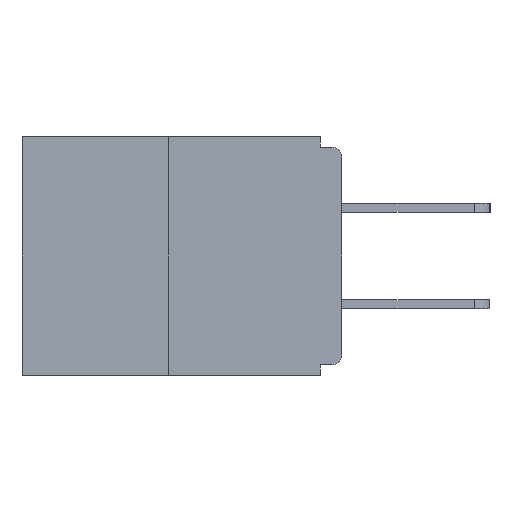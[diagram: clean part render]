
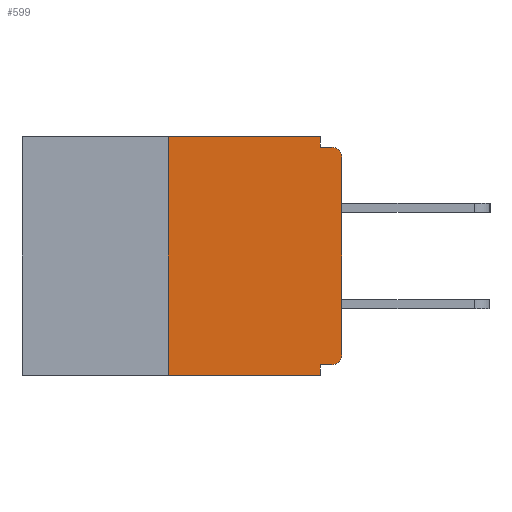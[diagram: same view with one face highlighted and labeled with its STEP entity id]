
A CAD part, left-side view. The second image highlights one B-rep face of the part: STEP entity #599.
In plain terms, the highlighted planar face has unit normal (-1, 0, 0).
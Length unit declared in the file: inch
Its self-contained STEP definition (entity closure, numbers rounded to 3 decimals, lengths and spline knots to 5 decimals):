
#55 = CARTESIAN_POINT ( 'NONE',  ( 0., 0.25, -0.343 ) ) ;
#145 = DIRECTION ( 'NONE',  ( 0., 0., -1. ) ) ;
#154 = LINE ( 'NONE', #9585, #1045 ) ;
#329 = CARTESIAN_POINT ( 'NONE',  ( 0., 0.031, -0.328 ) ) ;
#599 = ADVANCED_FACE ( 'NONE', ( #13697 ), #6927, .F. ) ;
#660 = CARTESIAN_POINT ( 'NONE',  ( 0., 0.031, -0.343 ) ) ;
#753 = CARTESIAN_POINT ( 'NONE',  ( 0., 0.031, 0. ) ) ;
#878 = CARTESIAN_POINT ( 'NONE',  ( 0., 0.015, -0.313 ) ) ;
#1045 = VECTOR ( 'NONE', #4793, 39.37008 ) ;
#1137 = VERTEX_POINT ( 'NONE', #2426 ) ;
#1263 = CIRCLE ( 'NONE', #7828, 0.015 ) ;
#1702 = CARTESIAN_POINT ( 'NONE',  ( 0., 0.25, 0. ) ) ;
#1756 = VECTOR ( 'NONE', #10959, 39.37008 ) ;
#1850 = DIRECTION ( 'NONE',  ( 0., -1., 0. ) ) ;
#2229 = CARTESIAN_POINT ( 'NONE',  ( 0., 0.46, 0. ) ) ;
#2411 = LINE ( 'NONE', #13906, #13651 ) ;
#2419 = DIRECTION ( 'NONE',  ( 1., 0., 0. ) ) ;
#2426 = CARTESIAN_POINT ( 'NONE',  ( 0., 0.015, -0.328 ) ) ;
#2439 = CARTESIAN_POINT ( 'NONE',  ( 0., 0., -0.03 ) ) ;
#2537 = EDGE_CURVE ( 'NONE', #13206, #12227, #7337, .T. ) ;
#2648 = ORIENTED_EDGE ( 'NONE', *, *, #13139, .F. ) ;
#2731 = CARTESIAN_POINT ( 'NONE',  ( 0., 0., -0.313 ) ) ;
#3042 = ORIENTED_EDGE ( 'NONE', *, *, #8581, .F. ) ;
#3074 = CARTESIAN_POINT ( 'NONE',  ( 0., 0.46, -0.343 ) ) ;
#3149 = LINE ( 'NONE', #2229, #14182 ) ;
#3300 = AXIS2_PLACEMENT_3D ( 'NONE', #878, #13658, #5589 ) ;
#3521 = LINE ( 'NONE', #8163, #3753 ) ;
#3753 = VECTOR ( 'NONE', #9519, 39.37008 ) ;
#4304 = CARTESIAN_POINT ( 'NONE',  ( 0., 0.25, 0. ) ) ;
#4618 = CARTESIAN_POINT ( 'NONE',  ( 0., 0.015, -0.015 ) ) ;
#4793 = DIRECTION ( 'NONE',  ( 0., 0., 1. ) ) ;
#5001 = VERTEX_POINT ( 'NONE', #10098 ) ;
#5079 = CARTESIAN_POINT ( 'NONE',  ( 0., 0.015, -0.03 ) ) ;
#5405 = ORIENTED_EDGE ( 'NONE', *, *, #7121, .F. ) ;
#5563 = CARTESIAN_POINT ( 'NONE',  ( 0., 0.031, 0. ) ) ;
#5589 = DIRECTION ( 'NONE',  ( 0., 0., -1. ) ) ;
#5591 = EDGE_CURVE ( 'NONE', #13206, #10536, #9686, .T. ) ;
#5718 = ORIENTED_EDGE ( 'NONE', *, *, #13248, .F. ) ;
#5751 = VERTEX_POINT ( 'NONE', #2439 ) ;
#6319 = CARTESIAN_POINT ( 'NONE',  ( 0., 0.031, -0.343 ) ) ;
#6501 = EDGE_CURVE ( 'NONE', #1137, #12887, #8638, .T. ) ;
#6508 = EDGE_LOOP ( 'NONE', ( #3042, #11984, #7573, #5718, #2648, #9656, #7468, #9655, #5405, #10322 ) ) ;
#6877 = VECTOR ( 'NONE', #12060, 39.37008 ) ;
#6927 = PLANE ( 'NONE',  #12223 ) ;
#7121 = EDGE_CURVE ( 'NONE', #5001, #11970, #3521, .T. ) ;
#7337 = LINE ( 'NONE', #1702, #6877 ) ;
#7468 = ORIENTED_EDGE ( 'NONE', *, *, #7993, .T. ) ;
#7477 = VECTOR ( 'NONE', #1850, 39.37008 ) ;
#7573 = ORIENTED_EDGE ( 'NONE', *, *, #5591, .T. ) ;
#7828 = AXIS2_PLACEMENT_3D ( 'NONE', #5079, #8427, #145 ) ;
#7834 = LINE ( 'NONE', #753, #13692 ) ;
#7993 = EDGE_CURVE ( 'NONE', #12887, #5751, #154, .T. ) ;
#8163 = CARTESIAN_POINT ( 'NONE',  ( 0., 0., -0.015 ) ) ;
#8427 = DIRECTION ( 'NONE',  ( -1., 0., 0. ) ) ;
#8581 = EDGE_CURVE ( 'NONE', #12227, #11376, #3149, .T. ) ;
#8638 = CIRCLE ( 'NONE', #3300, 0.015 ) ;
#9274 = DIRECTION ( 'NONE',  ( 0., 0., -1. ) ) ;
#9519 = DIRECTION ( 'NONE',  ( 0., -1., 0. ) ) ;
#9585 = CARTESIAN_POINT ( 'NONE',  ( 0., 0., 0. ) ) ;
#9655 = ORIENTED_EDGE ( 'NONE', *, *, #10407, .T. ) ;
#9656 = ORIENTED_EDGE ( 'NONE', *, *, #6501, .T. ) ;
#9678 = LINE ( 'NONE', #6319, #1756 ) ;
#9686 = LINE ( 'NONE', #3074, #7477 ) ;
#9902 = DIRECTION ( 'NONE',  ( 0., 0., -1. ) ) ;
#10098 = CARTESIAN_POINT ( 'NONE',  ( 0., 0.031, -0.015 ) ) ;
#10322 = ORIENTED_EDGE ( 'NONE', *, *, #14898, .F. ) ;
#10407 = EDGE_CURVE ( 'NONE', #5751, #11970, #1263, .T. ) ;
#10447 = DIRECTION ( 'NONE',  ( 0., -1., 0. ) ) ;
#10536 = VERTEX_POINT ( 'NONE', #660 ) ;
#10959 = DIRECTION ( 'NONE',  ( 0., 0., -1. ) ) ;
#11236 = VERTEX_POINT ( 'NONE', #329 ) ;
#11376 = VERTEX_POINT ( 'NONE', #5563 ) ;
#11559 = DIRECTION ( 'NONE',  ( 0., 1., 0. ) ) ;
#11970 = VERTEX_POINT ( 'NONE', #4618 ) ;
#11984 = ORIENTED_EDGE ( 'NONE', *, *, #2537, .F. ) ;
#12060 = DIRECTION ( 'NONE',  ( 0., 0., 1. ) ) ;
#12223 = AXIS2_PLACEMENT_3D ( 'NONE', #12784, #2419, #9274 ) ;
#12227 = VERTEX_POINT ( 'NONE', #4304 ) ;
#12784 = CARTESIAN_POINT ( 'NONE',  ( 0., 0.46, 0. ) ) ;
#12887 = VERTEX_POINT ( 'NONE', #2731 ) ;
#13139 = EDGE_CURVE ( 'NONE', #1137, #11236, #2411, .T. ) ;
#13206 = VERTEX_POINT ( 'NONE', #55 ) ;
#13248 = EDGE_CURVE ( 'NONE', #11236, #10536, #9678, .T. ) ;
#13651 = VECTOR ( 'NONE', #11559, 39.37008 ) ;
#13658 = DIRECTION ( 'NONE',  ( -1., 0., 0. ) ) ;
#13692 = VECTOR ( 'NONE', #9902, 39.37008 ) ;
#13697 = FACE_OUTER_BOUND ( 'NONE', #6508, .T. ) ;
#13906 = CARTESIAN_POINT ( 'NONE',  ( 0., 0., -0.328 ) ) ;
#14182 = VECTOR ( 'NONE', #10447, 39.37008 ) ;
#14898 = EDGE_CURVE ( 'NONE', #11376, #5001, #7834, .T. ) ;
